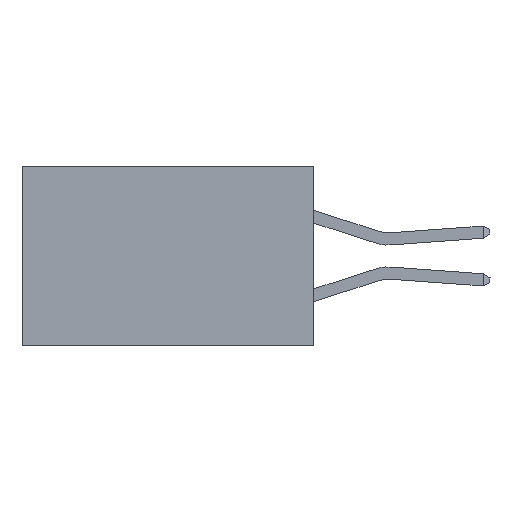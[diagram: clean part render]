
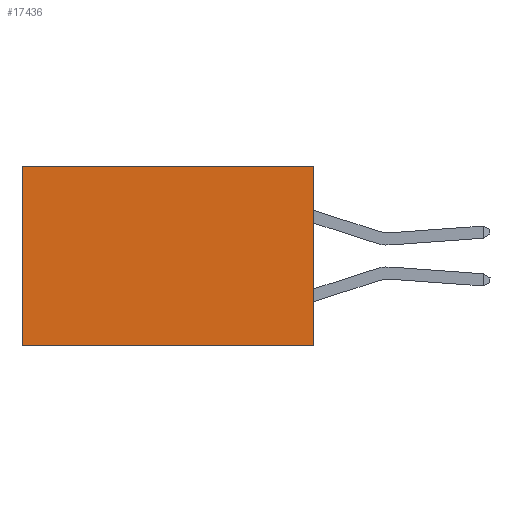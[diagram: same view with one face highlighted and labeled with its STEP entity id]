
A CAD part, left-side view. The second image highlights one B-rep face of the part: STEP entity #17436.
In plain terms, the highlighted planar face has unit normal (-1, 0, 0).
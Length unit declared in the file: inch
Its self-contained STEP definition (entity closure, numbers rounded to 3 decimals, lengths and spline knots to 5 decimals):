
#1097 = EDGE_CURVE ( 'NONE', #2441, #10769, #19517, .T. ) ;
#1261 = DIRECTION ( 'NONE',  ( 1., 0., 0. ) ) ;
#1464 = LINE ( 'NONE', #13748, #9941 ) ;
#2030 = DIRECTION ( 'NONE',  ( 0., 1., 0. ) ) ;
#2441 = VERTEX_POINT ( 'NONE', #3109 ) ;
#3109 = CARTESIAN_POINT ( 'NONE',  ( 0.2875, 0.6, 0. ) ) ;
#3830 = CARTESIAN_POINT ( 'NONE',  ( 0.2875, 0.6, 0. ) ) ;
#3909 = LINE ( 'NONE', #20402, #12309 ) ;
#4456 = VERTEX_POINT ( 'NONE', #15358 ) ;
#4585 = ORIENTED_EDGE ( 'NONE', *, *, #6092, .F. ) ;
#5059 = ORIENTED_EDGE ( 'NONE', *, *, #19241, .T. ) ;
#6054 = ORIENTED_EDGE ( 'NONE', *, *, #1097, .T. ) ;
#6092 = EDGE_CURVE ( 'NONE', #18961, #4456, #20522, .T. ) ;
#6513 = CARTESIAN_POINT ( 'NONE',  ( 0.2875, 0., 0. ) ) ;
#6772 = AXIS2_PLACEMENT_3D ( 'NONE', #11330, #1261, #12994 ) ;
#6867 = EDGE_CURVE ( 'NONE', #4456, #10769, #1464, .T. ) ;
#8038 = EDGE_LOOP ( 'NONE', ( #6054, #17705, #4585, #5059 ) ) ;
#9857 = CARTESIAN_POINT ( 'NONE',  ( 0.2875, 0., 0. ) ) ;
#9941 = VECTOR ( 'NONE', #2030, 39.37008 ) ;
#10769 = VERTEX_POINT ( 'NONE', #11645 ) ;
#11330 = CARTESIAN_POINT ( 'NONE',  ( 0.2875, 0., 0. ) ) ;
#11645 = CARTESIAN_POINT ( 'NONE',  ( 0.2875, 0.6, -0.37 ) ) ;
#12309 = VECTOR ( 'NONE', #15496, 39.37008 ) ;
#12994 = DIRECTION ( 'NONE',  ( 0., 0., -1. ) ) ;
#13748 = CARTESIAN_POINT ( 'NONE',  ( 0.2875, 0., -0.37 ) ) ;
#14571 = PLANE ( 'NONE',  #6772 ) ;
#14690 = DIRECTION ( 'NONE',  ( 0., 0., -1. ) ) ;
#15131 = VECTOR ( 'NONE', #14690, 39.37008 ) ;
#15358 = CARTESIAN_POINT ( 'NONE',  ( 0.2875, 0., -0.37 ) ) ;
#15496 = DIRECTION ( 'NONE',  ( 0., 1., 0. ) ) ;
#16397 = DIRECTION ( 'NONE',  ( 0., 0., -1. ) ) ;
#17436 = ADVANCED_FACE ( 'NONE', ( #19838 ), #14571, .F. ) ;
#17705 = ORIENTED_EDGE ( 'NONE', *, *, #6867, .F. ) ;
#18961 = VERTEX_POINT ( 'NONE', #9857 ) ;
#19241 = EDGE_CURVE ( 'NONE', #18961, #2441, #3909, .T. ) ;
#19517 = LINE ( 'NONE', #3830, #15131 ) ;
#19838 = FACE_OUTER_BOUND ( 'NONE', #8038, .T. ) ;
#19981 = VECTOR ( 'NONE', #16397, 39.37008 ) ;
#20402 = CARTESIAN_POINT ( 'NONE',  ( 0.2875, 0., 0. ) ) ;
#20522 = LINE ( 'NONE', #6513, #19981 ) ;
